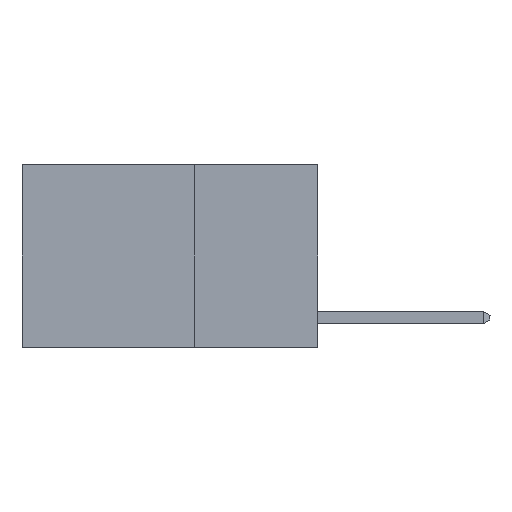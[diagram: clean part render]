
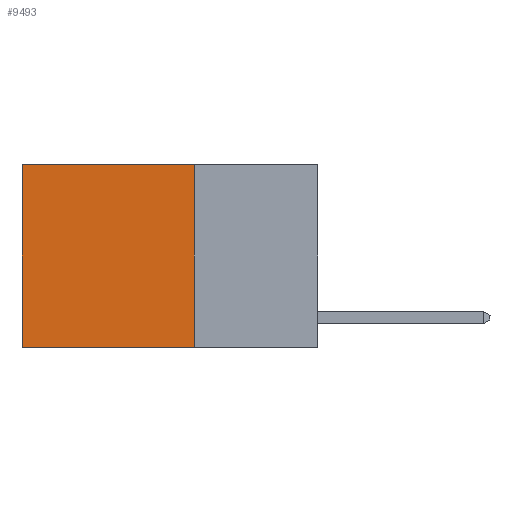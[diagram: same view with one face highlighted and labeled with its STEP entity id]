
A CAD part, left-side view. The second image highlights one B-rep face of the part: STEP entity #9493.
In plain terms, the highlighted planar face has unit normal (-1, 0, 0).
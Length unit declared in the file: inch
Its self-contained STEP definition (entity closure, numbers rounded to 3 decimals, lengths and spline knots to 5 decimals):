
#593 = EDGE_CURVE ( 'NONE', #20386, #15653, #11929, .T. ) ;
#1149 = DIRECTION ( 'NONE',  ( 1., 0., 0. ) ) ;
#2230 = CARTESIAN_POINT ( 'NONE',  ( 0.2625, 0.25, 0. ) ) ;
#3304 = VERTEX_POINT ( 'NONE', #8284 ) ;
#4376 = CARTESIAN_POINT ( 'NONE',  ( 0.2625, 0.25, 0. ) ) ;
#4893 = CARTESIAN_POINT ( 'NONE',  ( 0.2625, 0.25, 0. ) ) ;
#4909 = DIRECTION ( 'NONE',  ( 0., 0., -1. ) ) ;
#5879 = CARTESIAN_POINT ( 'NONE',  ( 0.2625, 0.25, -0.37 ) ) ;
#5994 = DIRECTION ( 'NONE',  ( 0., 0., -1. ) ) ;
#6933 = VERTEX_POINT ( 'NONE', #4893 ) ;
#7592 = EDGE_LOOP ( 'NONE', ( #10902, #19198, #9218, #14725 ) ) ;
#8284 = CARTESIAN_POINT ( 'NONE',  ( 0.2625, 0.6, 0. ) ) ;
#8460 = EDGE_CURVE ( 'NONE', #6933, #3304, #8637, .T. ) ;
#8637 = LINE ( 'NONE', #4376, #13619 ) ;
#8938 = CARTESIAN_POINT ( 'NONE',  ( 0.2625, 0.25, 0. ) ) ;
#9218 = ORIENTED_EDGE ( 'NONE', *, *, #21123, .F. ) ;
#9493 = ADVANCED_FACE ( 'NONE', ( #22620 ), #18851, .F. ) ;
#10432 = DIRECTION ( 'NONE',  ( 0., 1., 0. ) ) ;
#10902 = ORIENTED_EDGE ( 'NONE', *, *, #19786, .T. ) ;
#11929 = LINE ( 'NONE', #5879, #20194 ) ;
#12645 = LINE ( 'NONE', #22234, #21875 ) ;
#13114 = CARTESIAN_POINT ( 'NONE',  ( 0.2625, 0.25, -0.37 ) ) ;
#13619 = VECTOR ( 'NONE', #10432, 39.37008 ) ;
#14725 = ORIENTED_EDGE ( 'NONE', *, *, #8460, .T. ) ;
#15653 = VERTEX_POINT ( 'NONE', #24662 ) ;
#18851 = PLANE ( 'NONE',  #23169 ) ;
#19198 = ORIENTED_EDGE ( 'NONE', *, *, #593, .F. ) ;
#19786 = EDGE_CURVE ( 'NONE', #3304, #15653, #12645, .T. ) ;
#20190 = LINE ( 'NONE', #2230, #23170 ) ;
#20194 = VECTOR ( 'NONE', #23459, 39.37008 ) ;
#20386 = VERTEX_POINT ( 'NONE', #13114 ) ;
#20536 = DIRECTION ( 'NONE',  ( 0., 0., -1. ) ) ;
#21123 = EDGE_CURVE ( 'NONE', #6933, #20386, #20190, .T. ) ;
#21875 = VECTOR ( 'NONE', #20536, 39.37008 ) ;
#22234 = CARTESIAN_POINT ( 'NONE',  ( 0.2625, 0.6, 0. ) ) ;
#22620 = FACE_OUTER_BOUND ( 'NONE', #7592, .T. ) ;
#23169 = AXIS2_PLACEMENT_3D ( 'NONE', #8938, #1149, #4909 ) ;
#23170 = VECTOR ( 'NONE', #5994, 39.37008 ) ;
#23459 = DIRECTION ( 'NONE',  ( 0., 1., 0. ) ) ;
#24662 = CARTESIAN_POINT ( 'NONE',  ( 0.2625, 0.6, -0.37 ) ) ;
